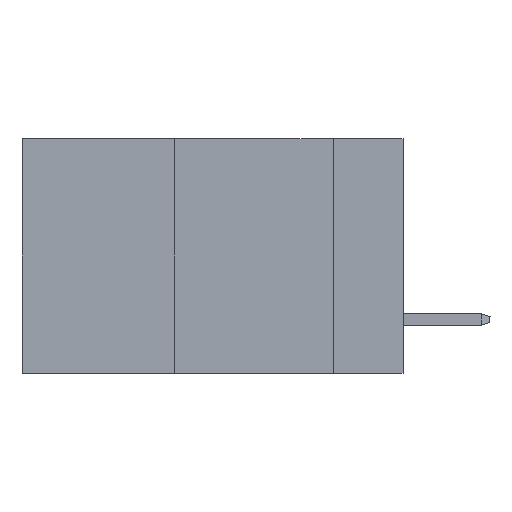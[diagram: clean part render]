
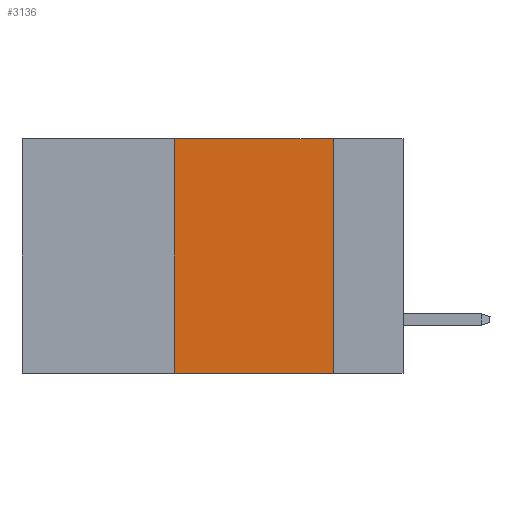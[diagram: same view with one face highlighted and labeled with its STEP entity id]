
A CAD part, left-side view. The second image highlights one B-rep face of the part: STEP entity #3136.
In plain terms, the highlighted planar face has unit normal (-1, 0, 0).
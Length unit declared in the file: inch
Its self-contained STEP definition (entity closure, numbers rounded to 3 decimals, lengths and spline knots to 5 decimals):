
#202 = DIRECTION ( 'NONE',  ( 0., 0., -1. ) ) ;
#1024 = ORIENTED_EDGE ( 'NONE', *, *, #7565, .F. ) ;
#1185 = DIRECTION ( 'NONE',  ( 0., -1., 0. ) ) ;
#1533 = CARTESIAN_POINT ( 'NONE',  ( 0., 0.6, 0. ) ) ;
#1885 = CARTESIAN_POINT ( 'NONE',  ( 0., 0.11, -0.37 ) ) ;
#1900 = DIRECTION ( 'NONE',  ( 0., -1., 0. ) ) ;
#2153 = AXIS2_PLACEMENT_3D ( 'NONE', #3305, #3198, #6509 ) ;
#2739 = VERTEX_POINT ( 'NONE', #4741 ) ;
#2923 = CARTESIAN_POINT ( 'NONE',  ( 0., 0.11, 0. ) ) ;
#3136 = ADVANCED_FACE ( 'NONE', ( #9729 ), #10655, .F. ) ;
#3198 = DIRECTION ( 'NONE',  ( 1., 0., 0. ) ) ;
#3305 = CARTESIAN_POINT ( 'NONE',  ( 0., 0.6, 0. ) ) ;
#3466 = ORIENTED_EDGE ( 'NONE', *, *, #8980, .F. ) ;
#3476 = VERTEX_POINT ( 'NONE', #10322 ) ;
#4542 = LINE ( 'NONE', #2923, #7081 ) ;
#4617 = VECTOR ( 'NONE', #1900, 39.37008 ) ;
#4741 = CARTESIAN_POINT ( 'NONE',  ( 0., 0.11, 0. ) ) ;
#5274 = LINE ( 'NONE', #6025, #9863 ) ;
#5630 = ORIENTED_EDGE ( 'NONE', *, *, #6689, .T. ) ;
#5690 = EDGE_LOOP ( 'NONE', ( #1024, #3466, #8049, #5630 ) ) ;
#5869 = VERTEX_POINT ( 'NONE', #1885 ) ;
#6025 = CARTESIAN_POINT ( 'NONE',  ( 0., 0.36, 0. ) ) ;
#6509 = DIRECTION ( 'NONE',  ( 0., 0., -1. ) ) ;
#6689 = EDGE_CURVE ( 'NONE', #9473, #5869, #6757, .T. ) ;
#6757 = LINE ( 'NONE', #7791, #4617 ) ;
#7081 = VECTOR ( 'NONE', #202, 39.37008 ) ;
#7565 = EDGE_CURVE ( 'NONE', #2739, #5869, #4542, .T. ) ;
#7791 = CARTESIAN_POINT ( 'NONE',  ( 0., 0.6, -0.37 ) ) ;
#8049 = ORIENTED_EDGE ( 'NONE', *, *, #8910, .F. ) ;
#8542 = DIRECTION ( 'NONE',  ( 0., 0., 1. ) ) ;
#8910 = EDGE_CURVE ( 'NONE', #9473, #3476, #5274, .T. ) ;
#8980 = EDGE_CURVE ( 'NONE', #3476, #2739, #9006, .T. ) ;
#9006 = LINE ( 'NONE', #1533, #10410 ) ;
#9473 = VERTEX_POINT ( 'NONE', #9747 ) ;
#9729 = FACE_OUTER_BOUND ( 'NONE', #5690, .T. ) ;
#9747 = CARTESIAN_POINT ( 'NONE',  ( 0., 0.36, -0.37 ) ) ;
#9863 = VECTOR ( 'NONE', #8542, 39.37008 ) ;
#10322 = CARTESIAN_POINT ( 'NONE',  ( 0., 0.36, 0. ) ) ;
#10410 = VECTOR ( 'NONE', #1185, 39.37008 ) ;
#10655 = PLANE ( 'NONE',  #2153 ) ;
